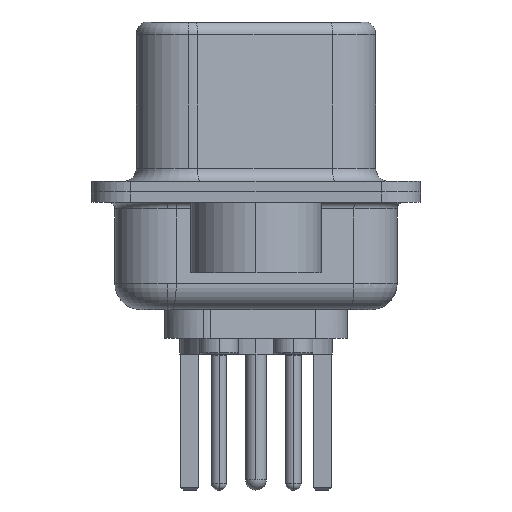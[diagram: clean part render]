
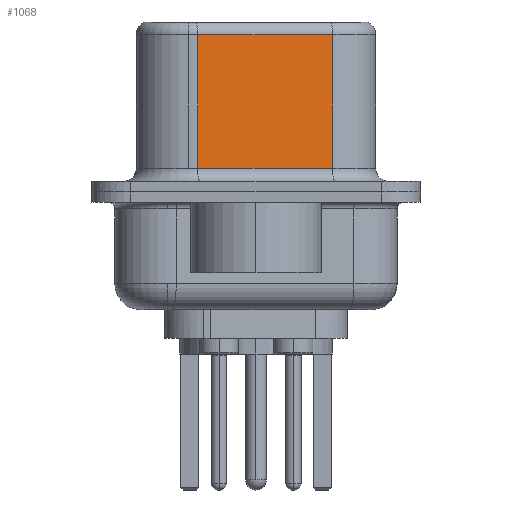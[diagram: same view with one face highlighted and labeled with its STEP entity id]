
A CAD part, left-side view. The second image highlights one B-rep face of the part: STEP entity #1068.
In plain terms, the highlighted planar face has unit normal (-0.985, -0.174, 0).
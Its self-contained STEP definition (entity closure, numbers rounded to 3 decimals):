
#781 = VECTOR ( 'NONE', #1216, 1000. ) ;
#1068 = ADVANCED_FACE ( 'NONE', ( #15558 ), #1633, .F. ) ;
#1216 = DIRECTION ( 'NONE',  ( 0., 0., -1. ) ) ;
#1564 = EDGE_CURVE ( 'NONE', #14713, #5616, #10619, .T. ) ;
#1633 = PLANE ( 'NONE',  #5872 ) ;
#2219 = DIRECTION ( 'NONE',  ( 0.174, -0.985, 0. ) ) ;
#3069 = EDGE_LOOP ( 'NONE', ( #10890, #10154, #14977, #9692 ) ) ;
#3448 = VERTEX_POINT ( 'NONE', #7673 ) ;
#4020 = LINE ( 'NONE', #6009, #10852 ) ;
#4096 = CARTESIAN_POINT ( 'NONE',  ( 4.58, -2.927, 6.02 ) ) ;
#4900 = EDGE_CURVE ( 'NONE', #14713, #13106, #11723, .T. ) ;
#5196 = VECTOR ( 'NONE', #12637, 1000. ) ;
#5359 = CARTESIAN_POINT ( 'NONE',  ( 4.58, -2.927, 6.52 ) ) ;
#5616 = VERTEX_POINT ( 'NONE', #8080 ) ;
#5872 = AXIS2_PLACEMENT_3D ( 'NONE', #12981, #10241, #15386 ) ;
#6009 = CARTESIAN_POINT ( 'NONE',  ( 4.58, -2.927, 0.9 ) ) ;
#7673 = CARTESIAN_POINT ( 'NONE',  ( 3.67, 2.233, 0.9 ) ) ;
#7879 = VECTOR ( 'NONE', #11783, 1000. ) ;
#8080 = CARTESIAN_POINT ( 'NONE',  ( 4.58, -2.927, 0.9 ) ) ;
#8265 = EDGE_CURVE ( 'NONE', #3448, #5616, #4020, .T. ) ;
#9692 = ORIENTED_EDGE ( 'NONE', *, *, #8265, .T. ) ;
#9841 = CARTESIAN_POINT ( 'NONE',  ( 3.67, 2.233, 6.02 ) ) ;
#10154 = ORIENTED_EDGE ( 'NONE', *, *, #4900, .T. ) ;
#10241 = DIRECTION ( 'NONE',  ( 0.985, 0.174, 0. ) ) ;
#10619 = LINE ( 'NONE', #5359, #781 ) ;
#10852 = VECTOR ( 'NONE', #2219, 1000. ) ;
#10890 = ORIENTED_EDGE ( 'NONE', *, *, #1564, .F. ) ;
#11202 = CARTESIAN_POINT ( 'NONE',  ( 4.58, -2.927, 6.02 ) ) ;
#11231 = LINE ( 'NONE', #12687, #5196 ) ;
#11723 = LINE ( 'NONE', #4096, #7879 ) ;
#11783 = DIRECTION ( 'NONE',  ( -0.174, 0.985, 0. ) ) ;
#12637 = DIRECTION ( 'NONE',  ( 0., 0., -1. ) ) ;
#12687 = CARTESIAN_POINT ( 'NONE',  ( 3.67, 2.233, 6.52 ) ) ;
#12981 = CARTESIAN_POINT ( 'NONE',  ( 4.58, -2.927, 6.52 ) ) ;
#13106 = VERTEX_POINT ( 'NONE', #9841 ) ;
#13634 = EDGE_CURVE ( 'NONE', #13106, #3448, #11231, .T. ) ;
#14713 = VERTEX_POINT ( 'NONE', #11202 ) ;
#14977 = ORIENTED_EDGE ( 'NONE', *, *, #13634, .T. ) ;
#15386 = DIRECTION ( 'NONE',  ( -0.174, 0.985, 0. ) ) ;
#15558 = FACE_OUTER_BOUND ( 'NONE', #3069, .T. ) ;
